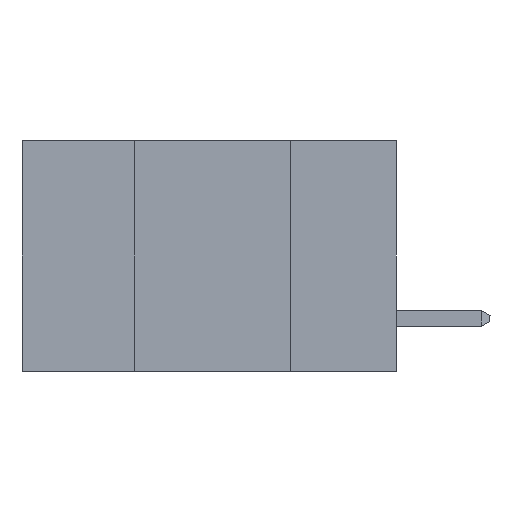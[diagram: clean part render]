
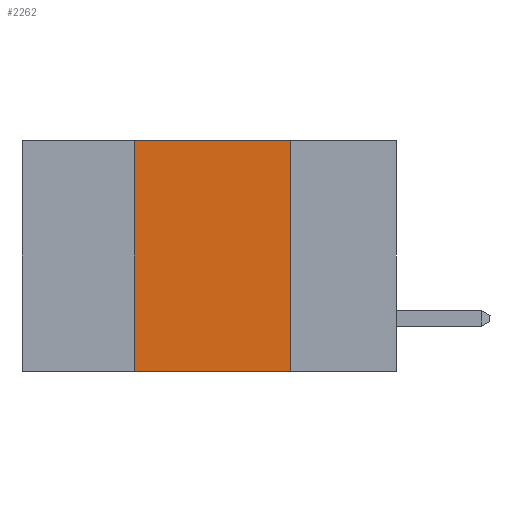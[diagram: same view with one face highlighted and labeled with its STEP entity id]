
A CAD part, left-side view. The second image highlights one B-rep face of the part: STEP entity #2262.
In plain terms, the highlighted planar face has unit normal (-1, 0, 0).
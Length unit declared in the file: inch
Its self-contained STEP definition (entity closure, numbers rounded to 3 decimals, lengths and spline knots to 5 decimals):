
#6 = VECTOR ( 'NONE', #8762, 39.37008 ) ;
#14 = VERTEX_POINT ( 'NONE', #6607 ) ;
#123 = DIRECTION ( 'NONE',  ( 0., 0., 1. ) ) ;
#163 = VERTEX_POINT ( 'NONE', #2865 ) ;
#410 = VECTOR ( 'NONE', #1455, 39.37008 ) ;
#440 = CARTESIAN_POINT ( 'NONE',  ( 0., 0.6, 0. ) ) ;
#551 = ORIENTED_EDGE ( 'NONE', *, *, #1779, .T. ) ;
#1037 = CARTESIAN_POINT ( 'NONE',  ( 0., 0.17, 0. ) ) ;
#1123 = LINE ( 'NONE', #3943, #6 ) ;
#1455 = DIRECTION ( 'NONE',  ( 0., 0., -1. ) ) ;
#1779 = EDGE_CURVE ( 'NONE', #4084, #163, #4688, .T. ) ;
#1807 = CARTESIAN_POINT ( 'NONE',  ( 0., 0.6, -0.37 ) ) ;
#1990 = LINE ( 'NONE', #4783, #3769 ) ;
#2047 = ORIENTED_EDGE ( 'NONE', *, *, #5859, .F. ) ;
#2092 = LINE ( 'NONE', #7639, #410 ) ;
#2262 = ADVANCED_FACE ( 'NONE', ( #6669 ), #5444, .F. ) ;
#2865 = CARTESIAN_POINT ( 'NONE',  ( 0., 0.17, -0.37 ) ) ;
#3008 = CARTESIAN_POINT ( 'NONE',  ( 0., 0.42, -0.37 ) ) ;
#3085 = EDGE_CURVE ( 'NONE', #6493, #163, #2092, .T. ) ;
#3202 = DIRECTION ( 'NONE',  ( 0., 0., -1. ) ) ;
#3464 = AXIS2_PLACEMENT_3D ( 'NONE', #440, #3933, #3202 ) ;
#3694 = ORIENTED_EDGE ( 'NONE', *, *, #3085, .F. ) ;
#3769 = VECTOR ( 'NONE', #123, 39.37008 ) ;
#3933 = DIRECTION ( 'NONE',  ( 1., 0., 0. ) ) ;
#3943 = CARTESIAN_POINT ( 'NONE',  ( 0., 0.6, 0. ) ) ;
#4084 = VERTEX_POINT ( 'NONE', #3008 ) ;
#4202 = VECTOR ( 'NONE', #7458, 39.37008 ) ;
#4550 = EDGE_CURVE ( 'NONE', #14, #6493, #1123, .T. ) ;
#4688 = LINE ( 'NONE', #1807, #4202 ) ;
#4783 = CARTESIAN_POINT ( 'NONE',  ( 0., 0.42, -0.37 ) ) ;
#5444 = PLANE ( 'NONE',  #3464 ) ;
#5859 = EDGE_CURVE ( 'NONE', #4084, #14, #1990, .T. ) ;
#6391 = ORIENTED_EDGE ( 'NONE', *, *, #4550, .F. ) ;
#6493 = VERTEX_POINT ( 'NONE', #1037 ) ;
#6527 = EDGE_LOOP ( 'NONE', ( #3694, #6391, #2047, #551 ) ) ;
#6607 = CARTESIAN_POINT ( 'NONE',  ( 0., 0.42, 0. ) ) ;
#6669 = FACE_OUTER_BOUND ( 'NONE', #6527, .T. ) ;
#7458 = DIRECTION ( 'NONE',  ( 0., -1., 0. ) ) ;
#7639 = CARTESIAN_POINT ( 'NONE',  ( 0., 0.17, -0.37 ) ) ;
#8762 = DIRECTION ( 'NONE',  ( 0., -1., 0. ) ) ;
